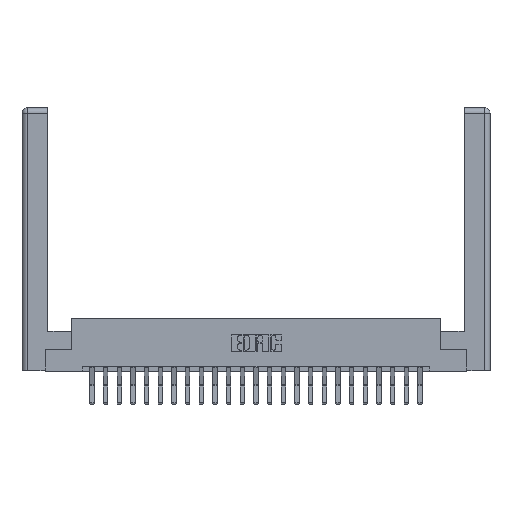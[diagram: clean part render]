
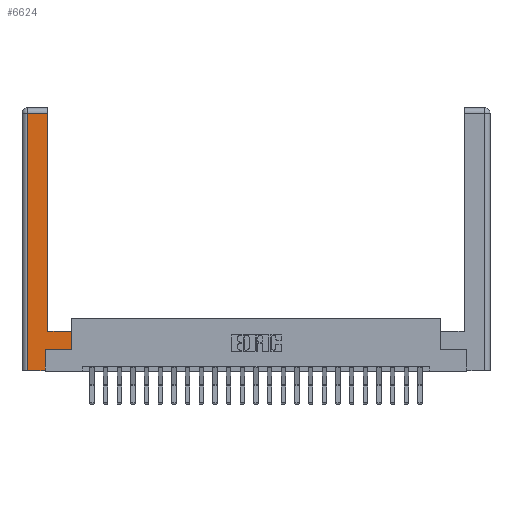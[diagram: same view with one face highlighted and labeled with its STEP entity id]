
A CAD part, top view. The second image highlights one B-rep face of the part: STEP entity #6624.
In plain terms, the highlighted planar face has unit normal (0, 0, 1).
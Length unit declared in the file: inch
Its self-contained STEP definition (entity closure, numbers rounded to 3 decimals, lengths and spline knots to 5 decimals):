
#549 = VERTEX_POINT ( 'NONE', #10581 ) ;
#1273 = CARTESIAN_POINT ( 'NONE',  ( 0.565, 0.245, 0. ) ) ;
#1620 = CARTESIAN_POINT ( 'NONE',  ( 0.565, 0.45, 0. ) ) ;
#2612 = LINE ( 'NONE', #16429, #20282 ) ;
#2697 = CARTESIAN_POINT ( 'NONE',  ( 0.265, 0., 0. ) ) ;
#2750 = VERTEX_POINT ( 'NONE', #11548 ) ;
#2923 = CARTESIAN_POINT ( 'NONE',  ( 0.265, 0.245, 0. ) ) ;
#3107 = ORIENTED_EDGE ( 'NONE', *, *, #3384, .T. ) ;
#3384 = EDGE_CURVE ( 'NONE', #549, #13770, #5638, .T. ) ;
#3499 = CARTESIAN_POINT ( 'NONE',  ( 0.295, 0.45, 0. ) ) ;
#4399 = VECTOR ( 'NONE', #21634, 39.37008 ) ;
#4411 = DIRECTION ( 'NONE',  ( -1., 0., 0. ) ) ;
#4614 = DIRECTION ( 'NONE',  ( 1., 0., 0. ) ) ;
#4779 = VERTEX_POINT ( 'NONE', #22877 ) ;
#5234 = VERTEX_POINT ( 'NONE', #16256 ) ;
#5638 = LINE ( 'NONE', #20986, #10024 ) ;
#6059 = EDGE_CURVE ( 'NONE', #2750, #4779, #6389, .T. ) ;
#6389 = LINE ( 'NONE', #2923, #11684 ) ;
#6624 = ADVANCED_FACE ( 'NONE', ( #23355 ), #9683, .F. ) ;
#6877 = LINE ( 'NONE', #2697, #15672 ) ;
#7015 = VECTOR ( 'NONE', #14968, 39.37008 ) ;
#7171 = DIRECTION ( 'NONE',  ( 0., 1., 0. ) ) ;
#7684 = VECTOR ( 'NONE', #4411, 39.37008 ) ;
#7786 = DIRECTION ( 'NONE',  ( -1., 0., 0. ) ) ;
#9652 = DIRECTION ( 'NONE',  ( -1., 0., 0. ) ) ;
#9663 = DIRECTION ( 'NONE',  ( 0., -1., 0. ) ) ;
#9683 = PLANE ( 'NONE',  #12791 ) ;
#10024 = VECTOR ( 'NONE', #9663, 39.37008 ) ;
#10429 = ORIENTED_EDGE ( 'NONE', *, *, #23155, .T. ) ;
#10581 = CARTESIAN_POINT ( 'NONE',  ( 0.0615, 2.94, 0. ) ) ;
#10937 = ORIENTED_EDGE ( 'NONE', *, *, #6059, .T. ) ;
#11064 = CARTESIAN_POINT ( 'NONE',  ( 0.565, 0.245, 0. ) ) ;
#11299 = VERTEX_POINT ( 'NONE', #1273 ) ;
#11548 = CARTESIAN_POINT ( 'NONE',  ( 0.265, 0., 0. ) ) ;
#11684 = VECTOR ( 'NONE', #16058, 39.37008 ) ;
#11723 = CARTESIAN_POINT ( 'NONE',  ( 0., 0., 0. ) ) ;
#12223 = CARTESIAN_POINT ( 'NONE',  ( 0.295, 3., 0. ) ) ;
#12657 = EDGE_CURVE ( 'NONE', #13276, #16471, #12689, .T. ) ;
#12689 = LINE ( 'NONE', #17464, #7684 ) ;
#12791 = AXIS2_PLACEMENT_3D ( 'NONE', #11723, #13624, #7786 ) ;
#13276 = VERTEX_POINT ( 'NONE', #1620 ) ;
#13300 = ORIENTED_EDGE ( 'NONE', *, *, #17420, .T. ) ;
#13624 = DIRECTION ( 'NONE',  ( 0., 0., -1. ) ) ;
#13770 = VERTEX_POINT ( 'NONE', #16827 ) ;
#14968 = DIRECTION ( 'NONE',  ( 1., 0., 0. ) ) ;
#15101 = EDGE_CURVE ( 'NONE', #13770, #2750, #6877, .T. ) ;
#15353 = EDGE_CURVE ( 'NONE', #5234, #549, #17170, .T. ) ;
#15672 = VECTOR ( 'NONE', #4614, 39.37008 ) ;
#16058 = DIRECTION ( 'NONE',  ( 0., 1., 0. ) ) ;
#16256 = CARTESIAN_POINT ( 'NONE',  ( 0.295, 2.94, 0. ) ) ;
#16429 = CARTESIAN_POINT ( 'NONE',  ( 0.565, 0.45, 0. ) ) ;
#16471 = VERTEX_POINT ( 'NONE', #3499 ) ;
#16827 = CARTESIAN_POINT ( 'NONE',  ( 0.0615, 0., 0. ) ) ;
#17170 = LINE ( 'NONE', #17429, #18940 ) ;
#17420 = EDGE_CURVE ( 'NONE', #11299, #13276, #2612, .T. ) ;
#17429 = CARTESIAN_POINT ( 'NONE',  ( 0.0615, 2.94, 0. ) ) ;
#17464 = CARTESIAN_POINT ( 'NONE',  ( 0.295, 0.45, 0. ) ) ;
#18414 = EDGE_CURVE ( 'NONE', #16471, #5234, #19399, .T. ) ;
#18940 = VECTOR ( 'NONE', #9652, 39.37008 ) ;
#19399 = LINE ( 'NONE', #12223, #4399 ) ;
#20282 = VECTOR ( 'NONE', #7171, 39.37008 ) ;
#20832 = ORIENTED_EDGE ( 'NONE', *, *, #18414, .T. ) ;
#20960 = EDGE_LOOP ( 'NONE', ( #20832, #21951, #3107, #21120, #10937, #10429, #13300, #21601 ) ) ;
#20986 = CARTESIAN_POINT ( 'NONE',  ( 0.0615, 0., 0. ) ) ;
#21120 = ORIENTED_EDGE ( 'NONE', *, *, #15101, .T. ) ;
#21601 = ORIENTED_EDGE ( 'NONE', *, *, #12657, .T. ) ;
#21634 = DIRECTION ( 'NONE',  ( 0., 1., 0. ) ) ;
#21951 = ORIENTED_EDGE ( 'NONE', *, *, #15353, .T. ) ;
#22877 = CARTESIAN_POINT ( 'NONE',  ( 0.265, 0.245, 0. ) ) ;
#23155 = EDGE_CURVE ( 'NONE', #4779, #11299, #23756, .T. ) ;
#23355 = FACE_OUTER_BOUND ( 'NONE', #20960, .T. ) ;
#23756 = LINE ( 'NONE', #11064, #7015 ) ;
